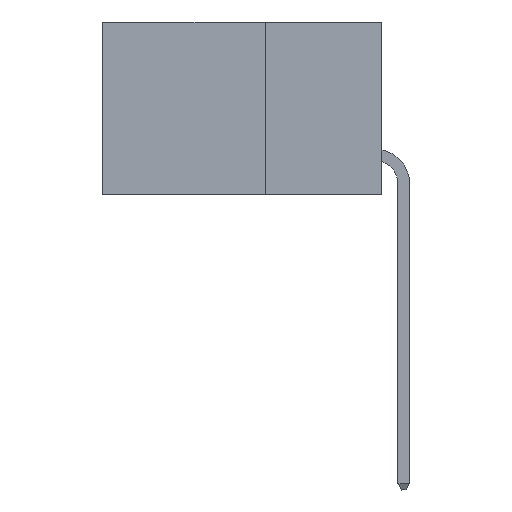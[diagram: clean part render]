
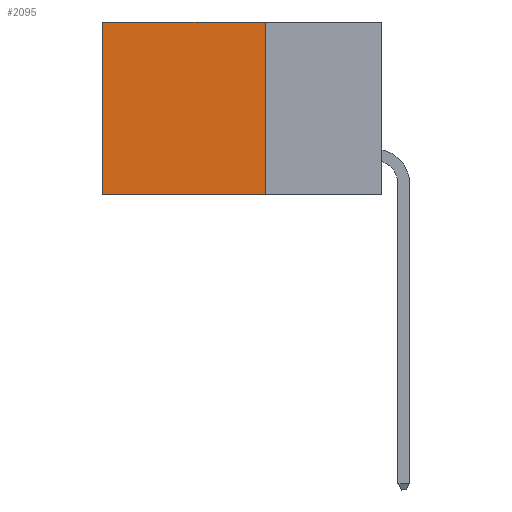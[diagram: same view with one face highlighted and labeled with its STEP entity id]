
A CAD part, left-side view. The second image highlights one B-rep face of the part: STEP entity #2095.
In plain terms, the highlighted planar face has unit normal (-1, 0, 0).
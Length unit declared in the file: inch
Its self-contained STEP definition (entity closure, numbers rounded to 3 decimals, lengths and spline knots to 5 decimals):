
#130 = DIRECTION ( 'NONE',  ( 0., 0., -1. ) ) ;
#267 = LINE ( 'NONE', #13805, #17335 ) ;
#602 = VECTOR ( 'NONE', #1192, 39.37008 ) ;
#1192 = DIRECTION ( 'NONE',  ( 0., 1., 0. ) ) ;
#2095 = ADVANCED_FACE ( 'NONE', ( #18980 ), #15129, .F. ) ;
#2319 = EDGE_CURVE ( 'NONE', #19137, #13542, #8718, .T. ) ;
#2367 = VERTEX_POINT ( 'NONE', #5347 ) ;
#2664 = EDGE_CURVE ( 'NONE', #13542, #14594, #267, .T. ) ;
#4871 = DIRECTION ( 'NONE',  ( 0., 0., -1. ) ) ;
#4940 = DIRECTION ( 'NONE',  ( 1., 0., 0. ) ) ;
#4944 = EDGE_LOOP ( 'NONE', ( #14790, #13736, #15635, #18637 ) ) ;
#5347 = CARTESIAN_POINT ( 'NONE',  ( 0.2875, 0.6, 0. ) ) ;
#7145 = CARTESIAN_POINT ( 'NONE',  ( 0.2875, 0.6, 0. ) ) ;
#7485 = AXIS2_PLACEMENT_3D ( 'NONE', #11823, #4940, #4871 ) ;
#8643 = DIRECTION ( 'NONE',  ( 0., 1., 0. ) ) ;
#8718 = LINE ( 'NONE', #17689, #19499 ) ;
#10126 = LINE ( 'NONE', #14944, #602 ) ;
#10158 = VECTOR ( 'NONE', #20826, 39.37008 ) ;
#11823 = CARTESIAN_POINT ( 'NONE',  ( 0.2875, 0.25, 0. ) ) ;
#11984 = EDGE_CURVE ( 'NONE', #2367, #14594, #14787, .T. ) ;
#12505 = CARTESIAN_POINT ( 'NONE',  ( 0.2875, 0.25, -0.37 ) ) ;
#13542 = VERTEX_POINT ( 'NONE', #12505 ) ;
#13736 = ORIENTED_EDGE ( 'NONE', *, *, #2664, .F. ) ;
#13805 = CARTESIAN_POINT ( 'NONE',  ( 0.2875, 0.25, -0.37 ) ) ;
#14594 = VERTEX_POINT ( 'NONE', #19973 ) ;
#14787 = LINE ( 'NONE', #7145, #10158 ) ;
#14790 = ORIENTED_EDGE ( 'NONE', *, *, #11984, .T. ) ;
#14944 = CARTESIAN_POINT ( 'NONE',  ( 0.2875, 0.25, 0. ) ) ;
#15129 = PLANE ( 'NONE',  #7485 ) ;
#15635 = ORIENTED_EDGE ( 'NONE', *, *, #2319, .F. ) ;
#16970 = EDGE_CURVE ( 'NONE', #19137, #2367, #10126, .T. ) ;
#17335 = VECTOR ( 'NONE', #8643, 39.37008 ) ;
#17689 = CARTESIAN_POINT ( 'NONE',  ( 0.2875, 0.25, 0. ) ) ;
#18637 = ORIENTED_EDGE ( 'NONE', *, *, #16970, .T. ) ;
#18980 = FACE_OUTER_BOUND ( 'NONE', #4944, .T. ) ;
#19137 = VERTEX_POINT ( 'NONE', #20570 ) ;
#19499 = VECTOR ( 'NONE', #130, 39.37008 ) ;
#19973 = CARTESIAN_POINT ( 'NONE',  ( 0.2875, 0.6, -0.37 ) ) ;
#20570 = CARTESIAN_POINT ( 'NONE',  ( 0.2875, 0.25, 0. ) ) ;
#20826 = DIRECTION ( 'NONE',  ( 0., 0., -1. ) ) ;
